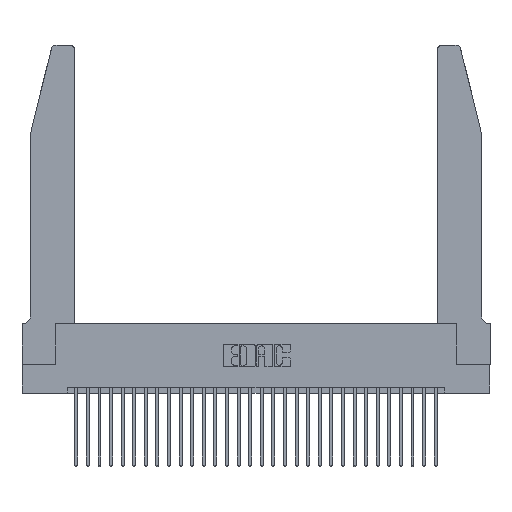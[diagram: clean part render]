
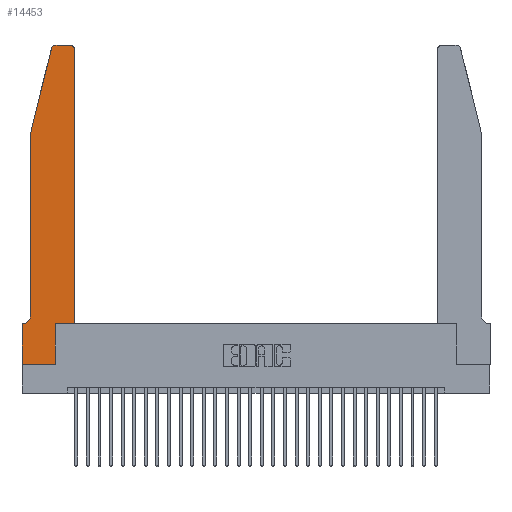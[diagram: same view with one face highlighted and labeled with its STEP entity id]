
A CAD part, top view. The second image highlights one B-rep face of the part: STEP entity #14453.
In plain terms, the highlighted planar face has unit normal (0, 0, 1).
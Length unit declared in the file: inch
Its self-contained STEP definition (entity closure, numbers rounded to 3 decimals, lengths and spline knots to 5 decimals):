
#182 = DIRECTION ( 'NONE',  ( 0., 0., -1. ) ) ;
#433 = VECTOR ( 'NONE', #16679, 39.37008 ) ;
#763 = EDGE_CURVE ( 'NONE', #14469, #17637, #19797, .T. ) ;
#908 = CARTESIAN_POINT ( 'NONE',  ( 0.0055, 0.35, 0.37 ) ) ;
#1024 = CARTESIAN_POINT ( 'NONE',  ( 0.4205, 2.72, 0.37 ) ) ;
#1875 = EDGE_CURVE ( 'NONE', #24054, #14469, #27802, .T. ) ;
#1888 = VERTEX_POINT ( 'NONE', #23226 ) ;
#2120 = ORIENTED_EDGE ( 'NONE', *, *, #11156, .T. ) ;
#2193 = VECTOR ( 'NONE', #17752, 39.37008 ) ;
#2278 = DIRECTION ( 'NONE',  ( 1., 0., 0. ) ) ;
#2396 = VERTEX_POINT ( 'NONE', #20537 ) ;
#2442 = VERTEX_POINT ( 'NONE', #30067 ) ;
#2972 = CARTESIAN_POINT ( 'NONE',  ( 0.4205, 2.75, 0.37 ) ) ;
#3589 = DIRECTION ( 'NONE',  ( 1., 0., 0. ) ) ;
#4221 = LINE ( 'NONE', #19192, #16440 ) ;
#4897 = EDGE_CURVE ( 'NONE', #9611, #8853, #21580, .T. ) ;
#5030 = ORIENTED_EDGE ( 'NONE', *, *, #16895, .T. ) ;
#5851 = EDGE_CURVE ( 'NONE', #12416, #2442, #20796, .T. ) ;
#6438 = DIRECTION ( 'NONE',  ( 0., -1., 0. ) ) ;
#6536 = LINE ( 'NONE', #22641, #31127 ) ;
#6838 = ORIENTED_EDGE ( 'NONE', *, *, #763, .T. ) ;
#7766 = EDGE_CURVE ( 'NONE', #8853, #2396, #23291, .T. ) ;
#8498 = VERTEX_POINT ( 'NONE', #23663 ) ;
#8573 = CARTESIAN_POINT ( 'NONE',  ( 0., 0.35, 0.37 ) ) ;
#8680 = AXIS2_PLACEMENT_3D ( 'NONE', #22199, #182, #18923 ) ;
#8838 = EDGE_LOOP ( 'NONE', ( #29204, #17864, #2120, #13046, #6838, #27355, #5030, #29345, #20719, #9873, #15449, #13982 ) ) ;
#8853 = VERTEX_POINT ( 'NONE', #27159 ) ;
#8856 = VECTOR ( 'NONE', #6438, 39.37008 ) ;
#9581 = VECTOR ( 'NONE', #12906, 39.37008 ) ;
#9611 = VERTEX_POINT ( 'NONE', #29594 ) ;
#9873 = ORIENTED_EDGE ( 'NONE', *, *, #29681, .T. ) ;
#10048 = VERTEX_POINT ( 'NONE', #2972 ) ;
#10426 = CARTESIAN_POINT ( 'NONE',  ( 0.0755, 0.35, 0.37 ) ) ;
#11071 = PLANE ( 'NONE',  #17099 ) ;
#11156 = EDGE_CURVE ( 'NONE', #2442, #24054, #13079, .T. ) ;
#12416 = VERTEX_POINT ( 'NONE', #19551 ) ;
#12906 = DIRECTION ( 'NONE',  ( -1., 0., 0. ) ) ;
#12916 = VECTOR ( 'NONE', #18345, 39.37008 ) ;
#12982 = EDGE_CURVE ( 'NONE', #10048, #12416, #19972, .T. ) ;
#13046 = ORIENTED_EDGE ( 'NONE', *, *, #1875, .T. ) ;
#13079 = LINE ( 'NONE', #28236, #24857 ) ;
#13982 = ORIENTED_EDGE ( 'NONE', *, *, #21001, .T. ) ;
#14453 = ADVANCED_FACE ( 'NONE', ( #18078 ), #11071, .T. ) ;
#14469 = VERTEX_POINT ( 'NONE', #27594 ) ;
#15124 = LINE ( 'NONE', #15993, #12916 ) ;
#15375 = CARTESIAN_POINT ( 'NONE',  ( 0., 0., 0.37 ) ) ;
#15449 = ORIENTED_EDGE ( 'NONE', *, *, #23943, .T. ) ;
#15874 = DIRECTION ( 'NONE',  ( 1., 0., 0. ) ) ;
#15993 = CARTESIAN_POINT ( 'NONE',  ( 0.4505, 0.35, 0.37 ) ) ;
#16440 = VECTOR ( 'NONE', #21558, 39.37008 ) ;
#16679 = DIRECTION ( 'NONE',  ( -1., 0., 0. ) ) ;
#16895 = EDGE_CURVE ( 'NONE', #17251, #9611, #6536, .T. ) ;
#16983 = DIRECTION ( 'NONE',  ( 0., 0., 1. ) ) ;
#17099 = AXIS2_PLACEMENT_3D ( 'NONE', #8573, #29963, #15874 ) ;
#17251 = VERTEX_POINT ( 'NONE', #19121 ) ;
#17637 = VERTEX_POINT ( 'NONE', #908 ) ;
#17752 = DIRECTION ( 'NONE',  ( 1., 0., 0. ) ) ;
#17864 = ORIENTED_EDGE ( 'NONE', *, *, #5851, .T. ) ;
#18078 = FACE_OUTER_BOUND ( 'NONE', #8838, .T. ) ;
#18177 = DIRECTION ( 'NONE',  ( 0., 0., 1. ) ) ;
#18345 = DIRECTION ( 'NONE',  ( 0., 1., 0. ) ) ;
#18923 = DIRECTION ( 'NONE',  ( -1., 0., 0. ) ) ;
#19042 = CARTESIAN_POINT ( 'NONE',  ( 0.2605, 2.75, 0.37 ) ) ;
#19121 = CARTESIAN_POINT ( 'NONE',  ( 0., 0.35, 0.37 ) ) ;
#19192 = CARTESIAN_POINT ( 'NONE',  ( 0.4505, 0.35, 0.37 ) ) ;
#19551 = CARTESIAN_POINT ( 'NONE',  ( 0.284, 2.75, 0.37 ) ) ;
#19797 = CIRCLE ( 'NONE', #8680, 0.07 ) ;
#19972 = LINE ( 'NONE', #19042, #433 ) ;
#20537 = CARTESIAN_POINT ( 'NONE',  ( 0.2865, 0.35, 0.37 ) ) ;
#20633 = CIRCLE ( 'NONE', #30994, 0.03 ) ;
#20719 = ORIENTED_EDGE ( 'NONE', *, *, #7766, .T. ) ;
#20796 = CIRCLE ( 'NONE', #25321, 0.03 ) ;
#20875 = CARTESIAN_POINT ( 'NONE',  ( 0.0755, 2., 0.37 ) ) ;
#21001 = EDGE_CURVE ( 'NONE', #8498, #10048, #20633, .T. ) ;
#21558 = DIRECTION ( 'NONE',  ( 1., 0., 0. ) ) ;
#21580 = LINE ( 'NONE', #15375, #2193 ) ;
#22199 = CARTESIAN_POINT ( 'NONE',  ( 0.0055, 0.42, 0.37 ) ) ;
#22263 = LINE ( 'NONE', #10426, #9581 ) ;
#22641 = CARTESIAN_POINT ( 'NONE',  ( 0., 0., 0.37 ) ) ;
#23014 = CARTESIAN_POINT ( 'NONE',  ( 0.2865, 0.35, 0.37 ) ) ;
#23226 = CARTESIAN_POINT ( 'NONE',  ( 0.4505, 0.35, 0.37 ) ) ;
#23291 = LINE ( 'NONE', #23014, #28810 ) ;
#23595 = DIRECTION ( 'NONE',  ( -0.239, -0.971, 0. ) ) ;
#23663 = CARTESIAN_POINT ( 'NONE',  ( 0.4505, 2.72, 0.37 ) ) ;
#23943 = EDGE_CURVE ( 'NONE', #1888, #8498, #15124, .T. ) ;
#24054 = VERTEX_POINT ( 'NONE', #30862 ) ;
#24857 = VECTOR ( 'NONE', #23595, 39.37008 ) ;
#24987 = DIRECTION ( 'NONE',  ( 0., -1., 0. ) ) ;
#25321 = AXIS2_PLACEMENT_3D ( 'NONE', #31033, #16983, #2278 ) ;
#27159 = CARTESIAN_POINT ( 'NONE',  ( 0.2865, 0., 0.37 ) ) ;
#27355 = ORIENTED_EDGE ( 'NONE', *, *, #30824, .T. ) ;
#27594 = CARTESIAN_POINT ( 'NONE',  ( 0.0755, 0.42, 0.37 ) ) ;
#27802 = LINE ( 'NONE', #20875, #8856 ) ;
#28236 = CARTESIAN_POINT ( 'NONE',  ( 0.0755, 2., 0.37 ) ) ;
#28810 = VECTOR ( 'NONE', #30083, 39.37008 ) ;
#29204 = ORIENTED_EDGE ( 'NONE', *, *, #12982, .T. ) ;
#29345 = ORIENTED_EDGE ( 'NONE', *, *, #4897, .T. ) ;
#29594 = CARTESIAN_POINT ( 'NONE',  ( 0., 0., 0.37 ) ) ;
#29681 = EDGE_CURVE ( 'NONE', #2396, #1888, #4221, .T. ) ;
#29963 = DIRECTION ( 'NONE',  ( 0., 0., 1. ) ) ;
#30067 = CARTESIAN_POINT ( 'NONE',  ( 0.25487, 2.72718, 0.37 ) ) ;
#30083 = DIRECTION ( 'NONE',  ( 0., 1., 0. ) ) ;
#30824 = EDGE_CURVE ( 'NONE', #17637, #17251, #22263, .T. ) ;
#30862 = CARTESIAN_POINT ( 'NONE',  ( 0.0755, 2., 0.37 ) ) ;
#30994 = AXIS2_PLACEMENT_3D ( 'NONE', #1024, #18177, #3589 ) ;
#31033 = CARTESIAN_POINT ( 'NONE',  ( 0.284, 2.72, 0.37 ) ) ;
#31127 = VECTOR ( 'NONE', #24987, 39.37008 ) ;
